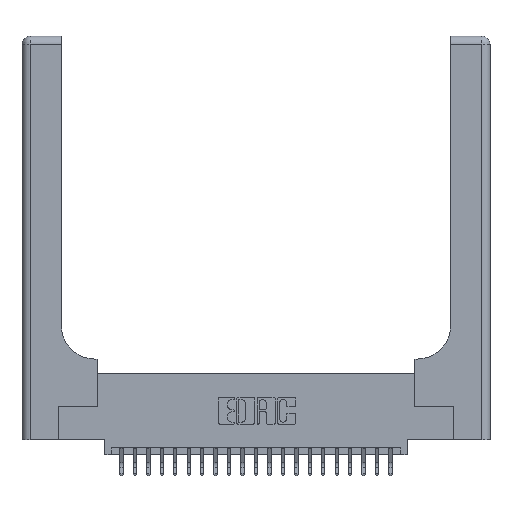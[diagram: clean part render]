
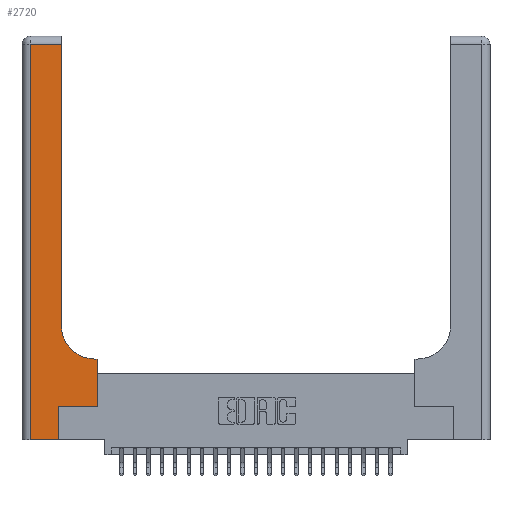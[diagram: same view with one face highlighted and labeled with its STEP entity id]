
A CAD part, top view. The second image highlights one B-rep face of the part: STEP entity #2720.
In plain terms, the highlighted planar face has unit normal (0, 0, 1).
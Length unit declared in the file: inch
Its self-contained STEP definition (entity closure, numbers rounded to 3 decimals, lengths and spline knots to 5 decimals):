
#321 = ORIENTED_EDGE ( 'NONE', *, *, #19136, .T. ) ;
#698 = LINE ( 'NONE', #7963, #10455 ) ;
#1269 = ORIENTED_EDGE ( 'NONE', *, *, #2995, .T. ) ;
#1353 = CARTESIAN_POINT ( 'NONE',  ( 0.5585, 0.25, 0.37 ) ) ;
#1585 = ORIENTED_EDGE ( 'NONE', *, *, #18124, .T. ) ;
#1654 = CARTESIAN_POINT ( 'NONE',  ( 0.269, 0., 0.37 ) ) ;
#1752 = DIRECTION ( 'NONE',  ( 1., 0., 0. ) ) ;
#1862 = ORIENTED_EDGE ( 'NONE', *, *, #2850, .T. ) ;
#2720 = ADVANCED_FACE ( 'NONE', ( #4004 ), #24305, .F. ) ;
#2835 = CARTESIAN_POINT ( 'NONE',  ( 0.5415, 0.85, 0.37 ) ) ;
#2850 = EDGE_CURVE ( 'NONE', #4119, #10903, #24574, .T. ) ;
#2923 = ORIENTED_EDGE ( 'NONE', *, *, #17331, .T. ) ;
#2995 = EDGE_CURVE ( 'NONE', #10903, #19209, #10935, .T. ) ;
#3080 = CARTESIAN_POINT ( 'NONE',  ( 0.06, 2.94, 0.37 ) ) ;
#3489 = CARTESIAN_POINT ( 'NONE',  ( 0.06, 0., 0.37 ) ) ;
#4004 = FACE_OUTER_BOUND ( 'NONE', #5484, .T. ) ;
#4119 = VERTEX_POINT ( 'NONE', #3489 ) ;
#4121 = CARTESIAN_POINT ( 'NONE',  ( 0.269, 0., 0.37 ) ) ;
#4294 = VECTOR ( 'NONE', #1752, 39.37008 ) ;
#4381 = VECTOR ( 'NONE', #20324, 39.37008 ) ;
#4773 = DIRECTION ( 'NONE',  ( 1., 0., 0. ) ) ;
#5186 = CARTESIAN_POINT ( 'NONE',  ( 0.2915, 2.94, 0.37 ) ) ;
#5248 = LINE ( 'NONE', #5997, #20481 ) ;
#5313 = DIRECTION ( 'NONE',  ( 0., 0., -1. ) ) ;
#5484 = EDGE_LOOP ( 'NONE', ( #10508, #2923, #1585, #1862, #1269, #321, #8373, #16995, #15309 ) ) ;
#5605 = LINE ( 'NONE', #8936, #4381 ) ;
#5668 = CARTESIAN_POINT ( 'NONE',  ( 0., 0., 0.37 ) ) ;
#5769 = CARTESIAN_POINT ( 'NONE',  ( 0.2915, 0.6, 0.37 ) ) ;
#5828 = VECTOR ( 'NONE', #6092, 39.37008 ) ;
#5864 = AXIS2_PLACEMENT_3D ( 'NONE', #22401, #5313, #18688 ) ;
#5936 = AXIS2_PLACEMENT_3D ( 'NONE', #2835, #16250, #4773 ) ;
#5997 = CARTESIAN_POINT ( 'NONE',  ( 0.269, 0.25, 0.37 ) ) ;
#6092 = DIRECTION ( 'NONE',  ( 0., 1., 0. ) ) ;
#7093 = LINE ( 'NONE', #1353, #12177 ) ;
#7963 = CARTESIAN_POINT ( 'NONE',  ( 0.06, 3., 0.37 ) ) ;
#8373 = ORIENTED_EDGE ( 'NONE', *, *, #19516, .T. ) ;
#8936 = CARTESIAN_POINT ( 'NONE',  ( 0.2915, 3., 0.37 ) ) ;
#8991 = VERTEX_POINT ( 'NONE', #11661 ) ;
#9359 = VERTEX_POINT ( 'NONE', #20344 ) ;
#10455 = VECTOR ( 'NONE', #13639, 39.37008 ) ;
#10508 = ORIENTED_EDGE ( 'NONE', *, *, #18413, .T. ) ;
#10903 = VERTEX_POINT ( 'NONE', #1654 ) ;
#10935 = LINE ( 'NONE', #4121, #5828 ) ;
#11636 = VECTOR ( 'NONE', #20367, 39.37008 ) ;
#11661 = CARTESIAN_POINT ( 'NONE',  ( 0.5415, 0.6, 0.37 ) ) ;
#12177 = VECTOR ( 'NONE', #24263, 39.37008 ) ;
#13608 = VECTOR ( 'NONE', #19107, 39.37008 ) ;
#13639 = DIRECTION ( 'NONE',  ( 0., -1., 0. ) ) ;
#14458 = CARTESIAN_POINT ( 'NONE',  ( 0.5585, 0.25, 0.37 ) ) ;
#15309 = ORIENTED_EDGE ( 'NONE', *, *, #21931, .T. ) ;
#16250 = DIRECTION ( 'NONE',  ( 0., 0., -1. ) ) ;
#16995 = ORIENTED_EDGE ( 'NONE', *, *, #24432, .T. ) ;
#17283 = VERTEX_POINT ( 'NONE', #3080 ) ;
#17331 = EDGE_CURVE ( 'NONE', #23849, #17283, #21705, .T. ) ;
#18124 = EDGE_CURVE ( 'NONE', #17283, #4119, #698, .T. ) ;
#18324 = VERTEX_POINT ( 'NONE', #14458 ) ;
#18413 = EDGE_CURVE ( 'NONE', #23387, #23849, #5605, .T. ) ;
#18457 = CARTESIAN_POINT ( 'NONE',  ( 0., 2.94, 0.37 ) ) ;
#18637 = LINE ( 'NONE', #5769, #13608 ) ;
#18688 = DIRECTION ( 'NONE',  ( -1., 0., 0. ) ) ;
#18997 = CARTESIAN_POINT ( 'NONE',  ( 0.2915, 0.85, 0.37 ) ) ;
#19107 = DIRECTION ( 'NONE',  ( -1., 0., 0. ) ) ;
#19136 = EDGE_CURVE ( 'NONE', #19209, #18324, #5248, .T. ) ;
#19165 = CIRCLE ( 'NONE', #5936, 0.25 ) ;
#19209 = VERTEX_POINT ( 'NONE', #23304 ) ;
#19516 = EDGE_CURVE ( 'NONE', #18324, #9359, #7093, .T. ) ;
#20324 = DIRECTION ( 'NONE',  ( 0., 1., 0. ) ) ;
#20344 = CARTESIAN_POINT ( 'NONE',  ( 0.5585, 0.6, 0.37 ) ) ;
#20367 = DIRECTION ( 'NONE',  ( -1., 0., 0. ) ) ;
#20481 = VECTOR ( 'NONE', #21219, 39.37008 ) ;
#21219 = DIRECTION ( 'NONE',  ( 1., 0., 0. ) ) ;
#21705 = LINE ( 'NONE', #18457, #11636 ) ;
#21931 = EDGE_CURVE ( 'NONE', #8991, #23387, #19165, .T. ) ;
#22401 = CARTESIAN_POINT ( 'NONE',  ( 0., 3., 0.37 ) ) ;
#23304 = CARTESIAN_POINT ( 'NONE',  ( 0.269, 0.25, 0.37 ) ) ;
#23387 = VERTEX_POINT ( 'NONE', #18997 ) ;
#23849 = VERTEX_POINT ( 'NONE', #5186 ) ;
#24263 = DIRECTION ( 'NONE',  ( 0., 1., 0. ) ) ;
#24305 = PLANE ( 'NONE',  #5864 ) ;
#24432 = EDGE_CURVE ( 'NONE', #9359, #8991, #18637, .T. ) ;
#24574 = LINE ( 'NONE', #5668, #4294 ) ;
